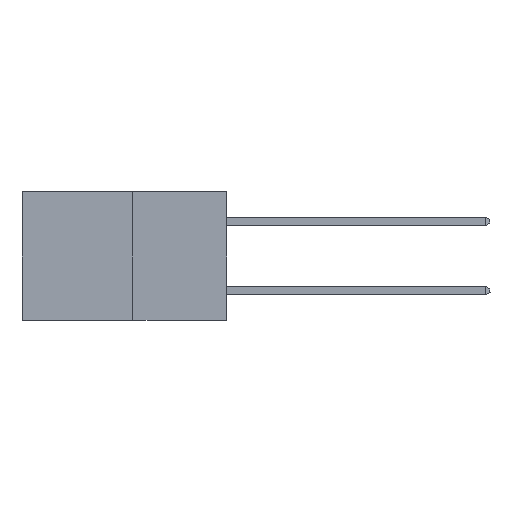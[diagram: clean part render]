
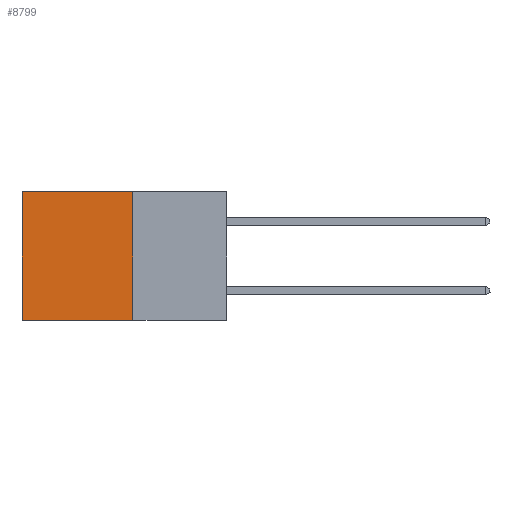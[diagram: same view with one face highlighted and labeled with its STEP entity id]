
A CAD part, left-side view. The second image highlights one B-rep face of the part: STEP entity #8799.
In plain terms, the highlighted planar face has unit normal (-1, 0, 0).
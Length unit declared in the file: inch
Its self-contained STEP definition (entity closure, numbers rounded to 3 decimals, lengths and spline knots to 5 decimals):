
#1962 = LINE ( 'NONE', #19969, #15939 ) ;
#2338 = CARTESIAN_POINT ( 'NONE',  ( 0.277, 0.27, -0.37 ) ) ;
#2787 = DIRECTION ( 'NONE',  ( 0., 0., -1. ) ) ;
#2992 = VERTEX_POINT ( 'NONE', #20671 ) ;
#3444 = ORIENTED_EDGE ( 'NONE', *, *, #8605, .T. ) ;
#3725 = DIRECTION ( 'NONE',  ( 0., 1., 0. ) ) ;
#4177 = DIRECTION ( 'NONE',  ( 0., 0., -1. ) ) ;
#4508 = CARTESIAN_POINT ( 'NONE',  ( 0.277, 0.27, -0.37 ) ) ;
#4948 = CARTESIAN_POINT ( 'NONE',  ( 0.277, 0.59, -0.37 ) ) ;
#6802 = EDGE_CURVE ( 'NONE', #8287, #21503, #17685, .T. ) ;
#7481 = CARTESIAN_POINT ( 'NONE',  ( 0.277, 0.27, -0.37 ) ) ;
#8287 = VERTEX_POINT ( 'NONE', #4508 ) ;
#8497 = ORIENTED_EDGE ( 'NONE', *, *, #6802, .F. ) ;
#8590 = VERTEX_POINT ( 'NONE', #23263 ) ;
#8594 = ORIENTED_EDGE ( 'NONE', *, *, #19269, .T. ) ;
#8605 = EDGE_CURVE ( 'NONE', #8590, #2992, #1962, .T. ) ;
#8799 = ADVANCED_FACE ( 'NONE', ( #12534 ), #18619, .F. ) ;
#9623 = LINE ( 'NONE', #10295, #18637 ) ;
#10295 = CARTESIAN_POINT ( 'NONE',  ( 0.277, 0.59, -0.37 ) ) ;
#10829 = ORIENTED_EDGE ( 'NONE', *, *, #23335, .F. ) ;
#10945 = VECTOR ( 'NONE', #20031, 39.37008 ) ;
#11934 = CARTESIAN_POINT ( 'NONE',  ( 0.277, 0.27, -0.37 ) ) ;
#12534 = FACE_OUTER_BOUND ( 'NONE', #16202, .T. ) ;
#15082 = DIRECTION ( 'NONE',  ( 1., 0., 0. ) ) ;
#15939 = VECTOR ( 'NONE', #3725, 39.37008 ) ;
#16049 = LINE ( 'NONE', #11934, #20809 ) ;
#16202 = EDGE_LOOP ( 'NONE', ( #8594, #8497, #10829, #3444 ) ) ;
#17685 = LINE ( 'NONE', #7481, #10945 ) ;
#18619 = PLANE ( 'NONE',  #20866 ) ;
#18637 = VECTOR ( 'NONE', #22888, 39.37008 ) ;
#19269 = EDGE_CURVE ( 'NONE', #2992, #21503, #9623, .T. ) ;
#19969 = CARTESIAN_POINT ( 'NONE',  ( 0.277, 0.27, 0. ) ) ;
#20031 = DIRECTION ( 'NONE',  ( 0., 1., 0. ) ) ;
#20671 = CARTESIAN_POINT ( 'NONE',  ( 0.277, 0.59, 0. ) ) ;
#20809 = VECTOR ( 'NONE', #2787, 39.37008 ) ;
#20866 = AXIS2_PLACEMENT_3D ( 'NONE', #2338, #15082, #4177 ) ;
#21503 = VERTEX_POINT ( 'NONE', #4948 ) ;
#22888 = DIRECTION ( 'NONE',  ( 0., 0., -1. ) ) ;
#23263 = CARTESIAN_POINT ( 'NONE',  ( 0.277, 0.27, 0. ) ) ;
#23335 = EDGE_CURVE ( 'NONE', #8590, #8287, #16049, .T. ) ;
